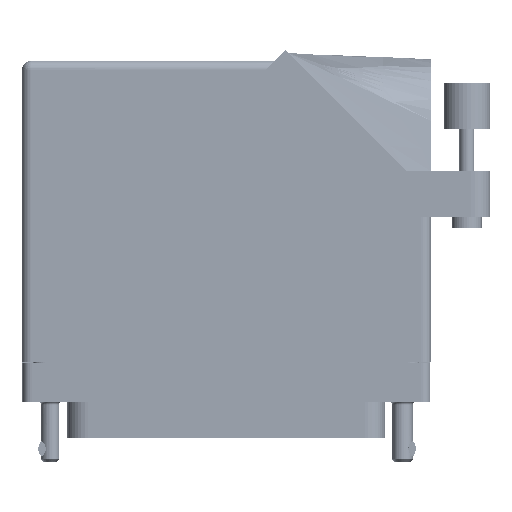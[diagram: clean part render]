
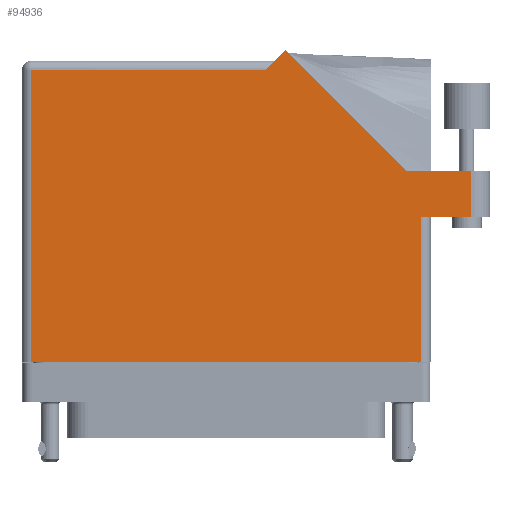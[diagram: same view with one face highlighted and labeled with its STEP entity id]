
A CAD part, front view. The second image highlights one B-rep face of the part: STEP entity #94936.
In plain terms, the highlighted face is planar.
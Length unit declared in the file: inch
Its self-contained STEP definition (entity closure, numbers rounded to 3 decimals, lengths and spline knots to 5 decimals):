
#580 = VERTEX_POINT ( 'NONE', #32278 ) ;
#2362 = ORIENTED_EDGE ( 'NONE', *, *, #29367, .T. ) ;
#2995 = DIRECTION ( 'NONE',  ( -1., 0., 0. ) ) ;
#5891 = VERTEX_POINT ( 'NONE', #97854 ) ;
#7429 = VERTEX_POINT ( 'NONE', #22707 ) ;
#8030 = DIRECTION ( 'NONE',  ( 0., 1., 0. ) ) ;
#8910 = DIRECTION ( 'NONE',  ( -1., 0., 0. ) ) ;
#9256 = LINE ( 'NONE', #49378, #94067 ) ;
#9896 = CARTESIAN_POINT ( 'NONE',  ( -1.3775, -0.1, 0.765 ) ) ;
#12589 = EDGE_CURVE ( 'NONE', #53935, #7429, #57325, .T. ) ;
#13763 = CARTESIAN_POINT ( 'NONE',  ( -1.3775, 1.868, 0.765 ) ) ;
#15004 = VERTEX_POINT ( 'NONE', #20609 ) ;
#15692 = FACE_OUTER_BOUND ( 'NONE', #99815, .T. ) ;
#19012 = VECTOR ( 'NONE', #36434, 39.37008 ) ;
#20609 = CARTESIAN_POINT ( 'NONE',  ( 1.6525, 1.187, 0.765 ) ) ;
#22241 = VECTOR ( 'NONE', #36311, 39.37008 ) ;
#22645 = LINE ( 'NONE', #86238, #49697 ) ;
#22707 = CARTESIAN_POINT ( 'NONE',  ( 1.3155, -0.1, 0.765 ) ) ;
#23290 = VECTOR ( 'NONE', #66665, 39.37008 ) ;
#24231 = VECTOR ( 'NONE', #2995, 39.37008 ) ;
#26529 = LINE ( 'NONE', #28065, #23290 ) ;
#27994 = CARTESIAN_POINT ( 'NONE',  ( 1.7775, 1.187, 0.765 ) ) ;
#28065 = CARTESIAN_POINT ( 'NONE',  ( 1.3775, 0.88, 0.765 ) ) ;
#29367 = EDGE_CURVE ( 'NONE', #96367, #74290, #26529, .T. ) ;
#30411 = AXIS2_PLACEMENT_3D ( 'NONE', #80345, #62617, #8910 ) ;
#30497 = LINE ( 'NONE', #62285, #81067 ) ;
#31311 = DIRECTION ( 'NONE',  ( 1., 0., 0. ) ) ;
#32025 = ORIENTED_EDGE ( 'NONE', *, *, #62394, .T. ) ;
#32278 = CARTESIAN_POINT ( 'NONE',  ( 0.2655, 1.868, 0.765 ) ) ;
#34992 = VECTOR ( 'NONE', #31311, 39.37008 ) ;
#36163 = EDGE_CURVE ( 'NONE', #7429, #96367, #52589, .T. ) ;
#36311 = DIRECTION ( 'NONE',  ( 0., -1., 0. ) ) ;
#36434 = DIRECTION ( 'NONE',  ( 0., 1., 0. ) ) ;
#41052 = DIRECTION ( 'NONE',  ( -0.707, -0.707, 0. ) ) ;
#45988 = ORIENTED_EDGE ( 'NONE', *, *, #36163, .T. ) ;
#46170 = EDGE_CURVE ( 'NONE', #49194, #580, #9256, .T. ) ;
#46199 = LINE ( 'NONE', #76449, #22241 ) ;
#47101 = DIRECTION ( 'NONE',  ( -1., 0., 0. ) ) ;
#48475 = ORIENTED_EDGE ( 'NONE', *, *, #12589, .T. ) ;
#48520 = PLANE ( 'NONE',  #30411 ) ;
#49194 = VERTEX_POINT ( 'NONE', #50223 ) ;
#49366 = VERTEX_POINT ( 'NONE', #74702 ) ;
#49378 = CARTESIAN_POINT ( 'NONE',  ( 0.3275, 1.93, 0.765 ) ) ;
#49697 = VECTOR ( 'NONE', #8030, 39.37008 ) ;
#50223 = CARTESIAN_POINT ( 'NONE',  ( 0.39821, 2.00071, 0.765 ) ) ;
#50696 = VECTOR ( 'NONE', #47101, 39.37008 ) ;
#52589 = LINE ( 'NONE', #67732, #19012 ) ;
#53369 = LINE ( 'NONE', #13763, #50696 ) ;
#53935 = VERTEX_POINT ( 'NONE', #99170 ) ;
#54210 = ORIENTED_EDGE ( 'NONE', *, *, #78274, .T. ) ;
#57325 = LINE ( 'NONE', #9896, #34992 ) ;
#60149 = ORIENTED_EDGE ( 'NONE', *, *, #46170, .T. ) ;
#61187 = ORIENTED_EDGE ( 'NONE', *, *, #91947, .T. ) ;
#62285 = CARTESIAN_POINT ( 'NONE',  ( 1.21192, 1.187, 0.765 ) ) ;
#62394 = EDGE_CURVE ( 'NONE', #5891, #49194, #30497, .T. ) ;
#62617 = DIRECTION ( 'NONE',  ( 0., 0., -1. ) ) ;
#64322 = EDGE_CURVE ( 'NONE', #74290, #15004, #22645, .T. ) ;
#65086 = CARTESIAN_POINT ( 'NONE',  ( 1.3155, 0.88, 0.765 ) ) ;
#66665 = DIRECTION ( 'NONE',  ( 1., 0., 0. ) ) ;
#67732 = CARTESIAN_POINT ( 'NONE',  ( 1.3155, 0.88, 0.765 ) ) ;
#74290 = VERTEX_POINT ( 'NONE', #79566 ) ;
#74702 = CARTESIAN_POINT ( 'NONE',  ( -1.3155, 1.868, 0.765 ) ) ;
#76449 = CARTESIAN_POINT ( 'NONE',  ( -1.3155, -0.1, 0.765 ) ) ;
#78274 = EDGE_CURVE ( 'NONE', #580, #49366, #53369, .T. ) ;
#79289 = EDGE_CURVE ( 'NONE', #15004, #5891, #97347, .T. ) ;
#79566 = CARTESIAN_POINT ( 'NONE',  ( 1.6525, 0.88, 0.765 ) ) ;
#80345 = CARTESIAN_POINT ( 'NONE',  ( -1.3775, 1.93, 0.765 ) ) ;
#81067 = VECTOR ( 'NONE', #86797, 39.37008 ) ;
#82660 = ORIENTED_EDGE ( 'NONE', *, *, #64322, .T. ) ;
#86238 = CARTESIAN_POINT ( 'NONE',  ( 1.6525, 1.187, 0.765 ) ) ;
#86797 = DIRECTION ( 'NONE',  ( -0.707, 0.707, 0. ) ) ;
#91947 = EDGE_CURVE ( 'NONE', #49366, #53935, #46199, .T. ) ;
#94067 = VECTOR ( 'NONE', #41052, 39.37008 ) ;
#94936 = ADVANCED_FACE ( 'NONE', ( #15692 ), #48520, .F. ) ;
#96367 = VERTEX_POINT ( 'NONE', #65086 ) ;
#96842 = ORIENTED_EDGE ( 'NONE', *, *, #79289, .T. ) ;
#97347 = LINE ( 'NONE', #27994, #24231 ) ;
#97854 = CARTESIAN_POINT ( 'NONE',  ( 1.21192, 1.187, 0.765 ) ) ;
#99170 = CARTESIAN_POINT ( 'NONE',  ( -1.3155, -0.1, 0.765 ) ) ;
#99815 = EDGE_LOOP ( 'NONE', ( #2362, #82660, #96842, #32025, #60149, #54210, #61187, #48475, #45988 ) ) ;
